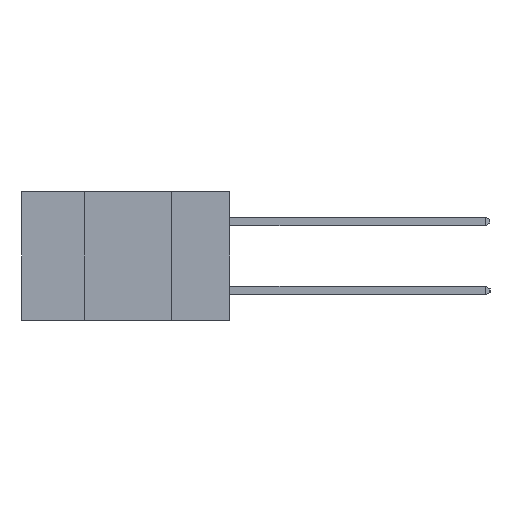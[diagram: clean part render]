
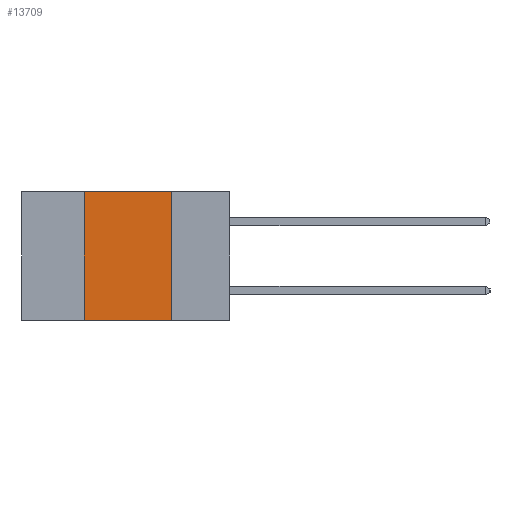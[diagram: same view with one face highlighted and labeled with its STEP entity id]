
A CAD part, left-side view. The second image highlights one B-rep face of the part: STEP entity #13709.
In plain terms, the highlighted planar face has unit normal (-1, 0, 0).
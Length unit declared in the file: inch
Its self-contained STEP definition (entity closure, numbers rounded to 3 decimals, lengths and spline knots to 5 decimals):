
#117 = CARTESIAN_POINT ( 'NONE',  ( 0., 0.6, 0. ) ) ;
#653 = ORIENTED_EDGE ( 'NONE', *, *, #7519, .F. ) ;
#672 = FACE_OUTER_BOUND ( 'NONE', #2943, .T. ) ;
#2353 = CARTESIAN_POINT ( 'NONE',  ( 0., 0.17, -0.37 ) ) ;
#2943 = EDGE_LOOP ( 'NONE', ( #653, #8196, #15302, #3517 ) ) ;
#2983 = DIRECTION ( 'NONE',  ( 0., 0., 1. ) ) ;
#3201 = VECTOR ( 'NONE', #2983, 39.37008 ) ;
#3517 = ORIENTED_EDGE ( 'NONE', *, *, #15006, .T. ) ;
#4055 = DIRECTION ( 'NONE',  ( 1., 0., 0. ) ) ;
#5406 = EDGE_CURVE ( 'NONE', #7683, #8955, #10255, .T. ) ;
#5512 = CARTESIAN_POINT ( 'NONE',  ( 0., 0.17, 0. ) ) ;
#6184 = CARTESIAN_POINT ( 'NONE',  ( 0., 0.42, -0.37 ) ) ;
#7519 = EDGE_CURVE ( 'NONE', #15474, #13472, #14562, .T. ) ;
#7648 = LINE ( 'NONE', #117, #10597 ) ;
#7683 = VERTEX_POINT ( 'NONE', #6184 ) ;
#7817 = EDGE_CURVE ( 'NONE', #8955, #15474, #7648, .T. ) ;
#7850 = CARTESIAN_POINT ( 'NONE',  ( 0., 0.42, 0. ) ) ;
#8196 = ORIENTED_EDGE ( 'NONE', *, *, #7817, .F. ) ;
#8394 = VECTOR ( 'NONE', #9672, 39.37008 ) ;
#8955 = VERTEX_POINT ( 'NONE', #7850 ) ;
#9616 = AXIS2_PLACEMENT_3D ( 'NONE', #11590, #4055, #12829 ) ;
#9672 = DIRECTION ( 'NONE',  ( 0., -1., 0. ) ) ;
#10248 = DIRECTION ( 'NONE',  ( 0., -1., 0. ) ) ;
#10255 = LINE ( 'NONE', #10481, #3201 ) ;
#10481 = CARTESIAN_POINT ( 'NONE',  ( 0., 0.42, -0.37 ) ) ;
#10597 = VECTOR ( 'NONE', #10248, 39.37008 ) ;
#11206 = VECTOR ( 'NONE', #13298, 39.37008 ) ;
#11590 = CARTESIAN_POINT ( 'NONE',  ( 0., 0.6, 0. ) ) ;
#11757 = LINE ( 'NONE', #14721, #8394 ) ;
#12829 = DIRECTION ( 'NONE',  ( 0., 0., -1. ) ) ;
#13298 = DIRECTION ( 'NONE',  ( 0., 0., -1. ) ) ;
#13365 = CARTESIAN_POINT ( 'NONE',  ( 0., 0.17, -0.37 ) ) ;
#13472 = VERTEX_POINT ( 'NONE', #2353 ) ;
#13709 = ADVANCED_FACE ( 'NONE', ( #672 ), #15326, .F. ) ;
#14562 = LINE ( 'NONE', #13365, #11206 ) ;
#14721 = CARTESIAN_POINT ( 'NONE',  ( 0., 0.6, -0.37 ) ) ;
#15006 = EDGE_CURVE ( 'NONE', #7683, #13472, #11757, .T. ) ;
#15302 = ORIENTED_EDGE ( 'NONE', *, *, #5406, .F. ) ;
#15326 = PLANE ( 'NONE',  #9616 ) ;
#15474 = VERTEX_POINT ( 'NONE', #5512 ) ;
